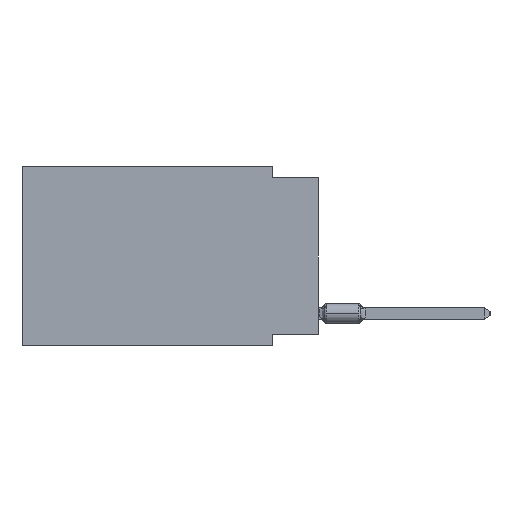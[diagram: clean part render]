
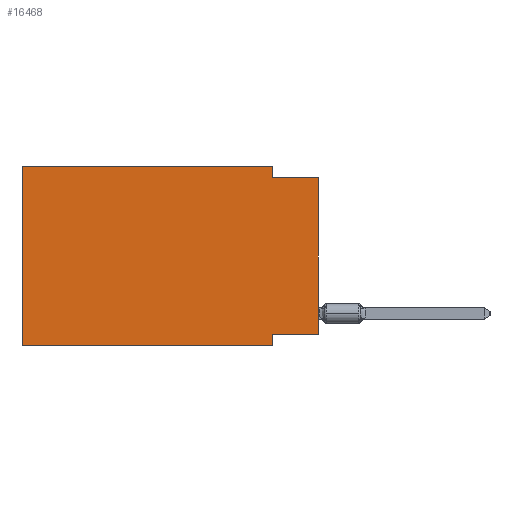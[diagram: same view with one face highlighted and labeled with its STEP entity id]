
A CAD part, left-side view. The second image highlights one B-rep face of the part: STEP entity #16468.
In plain terms, the highlighted planar face has unit normal (-1, 0, 0).
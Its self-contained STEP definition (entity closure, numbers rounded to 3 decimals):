
#1429 = ORIENTED_EDGE ( 'NONE', *, *, #13869, .F. ) ;
#1480 = EDGE_CURVE ( 'NONE', #26069, #17032, #21447, .T. ) ;
#1999 = FACE_OUTER_BOUND ( 'NONE', #13005, .T. ) ;
#2435 = DIRECTION ( 'NONE',  ( 0., 0., -1. ) ) ;
#2850 = EDGE_CURVE ( 'NONE', #8393, #25717, #11000, .T. ) ;
#3305 = ORIENTED_EDGE ( 'NONE', *, *, #23961, .F. ) ;
#3434 = CARTESIAN_POINT ( 'NONE',  ( 0., 0., -0.635 ) ) ;
#3687 = VERTEX_POINT ( 'NONE', #13850 ) ;
#4424 = ORIENTED_EDGE ( 'NONE', *, *, #1480, .T. ) ;
#4514 = CARTESIAN_POINT ( 'NONE',  ( 0., 16.383, 0. ) ) ;
#4655 = LINE ( 'NONE', #13677, #7923 ) ;
#4717 = CARTESIAN_POINT ( 'NONE',  ( 0., 16.383, -9.906 ) ) ;
#5050 = EDGE_CURVE ( 'NONE', #8393, #15261, #16560, .T. ) ;
#6239 = CARTESIAN_POINT ( 'NONE',  ( 0., 16.383, 0. ) ) ;
#6585 = CARTESIAN_POINT ( 'NONE',  ( 0., 2.54, -9.906 ) ) ;
#7616 = CARTESIAN_POINT ( 'NONE',  ( 0., 2.54, -9.906 ) ) ;
#7911 = DIRECTION ( 'NONE',  ( 0., 0., -1. ) ) ;
#7923 = VECTOR ( 'NONE', #20180, 1000. ) ;
#8393 = VERTEX_POINT ( 'NONE', #4717 ) ;
#8477 = VECTOR ( 'NONE', #15091, 1000. ) ;
#9090 = CARTESIAN_POINT ( 'NONE',  ( 0., 2.54, 0. ) ) ;
#9361 = ORIENTED_EDGE ( 'NONE', *, *, #5050, .T. ) ;
#9846 = DIRECTION ( 'NONE',  ( 0., -1., 0. ) ) ;
#10598 = VECTOR ( 'NONE', #10973, 1000. ) ;
#10973 = DIRECTION ( 'NONE',  ( 0., -1., 0. ) ) ;
#11000 = LINE ( 'NONE', #20175, #14948 ) ;
#11019 = PLANE ( 'NONE',  #20129 ) ;
#11770 = LINE ( 'NONE', #23294, #13088 ) ;
#12137 = VECTOR ( 'NONE', #23211, 1000. ) ;
#12884 = CARTESIAN_POINT ( 'NONE',  ( 0., 16.383, 0. ) ) ;
#13005 = EDGE_LOOP ( 'NONE', ( #4424, #24523, #22761, #1429, #28924, #9361, #3305, #16681 ) ) ;
#13088 = VECTOR ( 'NONE', #9846, 1000. ) ;
#13677 = CARTESIAN_POINT ( 'NONE',  ( 0., 0., -9.271 ) ) ;
#13850 = CARTESIAN_POINT ( 'NONE',  ( 0., 2.54, -0.635 ) ) ;
#13869 = EDGE_CURVE ( 'NONE', #25717, #18945, #17492, .T. ) ;
#14856 = LINE ( 'NONE', #7616, #19510 ) ;
#14948 = VECTOR ( 'NONE', #19595, 1000. ) ;
#15091 = DIRECTION ( 'NONE',  ( 0., 0., 1. ) ) ;
#15110 = VECTOR ( 'NONE', #24172, 1000. ) ;
#15261 = VERTEX_POINT ( 'NONE', #6585 ) ;
#15412 = CARTESIAN_POINT ( 'NONE',  ( 0., 2.54, -9.271 ) ) ;
#16468 = ADVANCED_FACE ( 'NONE', ( #1999 ), #11019, .F. ) ;
#16560 = LINE ( 'NONE', #28229, #12137 ) ;
#16681 = ORIENTED_EDGE ( 'NONE', *, *, #17456, .F. ) ;
#17032 = VERTEX_POINT ( 'NONE', #3434 ) ;
#17143 = CARTESIAN_POINT ( 'NONE',  ( 0., 0., -9.271 ) ) ;
#17363 = CARTESIAN_POINT ( 'NONE',  ( 0., 2.54, 0. ) ) ;
#17456 = EDGE_CURVE ( 'NONE', #26069, #28587, #4655, .T. ) ;
#17492 = LINE ( 'NONE', #6239, #10598 ) ;
#18945 = VERTEX_POINT ( 'NONE', #9090 ) ;
#19117 = EDGE_CURVE ( 'NONE', #18945, #3687, #28163, .T. ) ;
#19510 = VECTOR ( 'NONE', #7911, 1000. ) ;
#19595 = DIRECTION ( 'NONE',  ( 0., 0., 1. ) ) ;
#20129 = AXIS2_PLACEMENT_3D ( 'NONE', #4514, #24339, #2435 ) ;
#20175 = CARTESIAN_POINT ( 'NONE',  ( 0., 16.383, 0. ) ) ;
#20180 = DIRECTION ( 'NONE',  ( 0., 1., 0. ) ) ;
#20234 = EDGE_CURVE ( 'NONE', #3687, #17032, #11770, .T. ) ;
#21447 = LINE ( 'NONE', #21598, #8477 ) ;
#21598 = CARTESIAN_POINT ( 'NONE',  ( 0., 0., 0. ) ) ;
#22761 = ORIENTED_EDGE ( 'NONE', *, *, #19117, .F. ) ;
#23211 = DIRECTION ( 'NONE',  ( 0., -1., 0. ) ) ;
#23294 = CARTESIAN_POINT ( 'NONE',  ( 0., 0., -0.635 ) ) ;
#23961 = EDGE_CURVE ( 'NONE', #28587, #15261, #14856, .T. ) ;
#24172 = DIRECTION ( 'NONE',  ( 0., 0., -1. ) ) ;
#24339 = DIRECTION ( 'NONE',  ( 1., 0., 0. ) ) ;
#24523 = ORIENTED_EDGE ( 'NONE', *, *, #20234, .F. ) ;
#25717 = VERTEX_POINT ( 'NONE', #12884 ) ;
#26069 = VERTEX_POINT ( 'NONE', #17143 ) ;
#28163 = LINE ( 'NONE', #17363, #15110 ) ;
#28229 = CARTESIAN_POINT ( 'NONE',  ( 0., 16.383, -9.906 ) ) ;
#28587 = VERTEX_POINT ( 'NONE', #15412 ) ;
#28924 = ORIENTED_EDGE ( 'NONE', *, *, #2850, .F. ) ;
